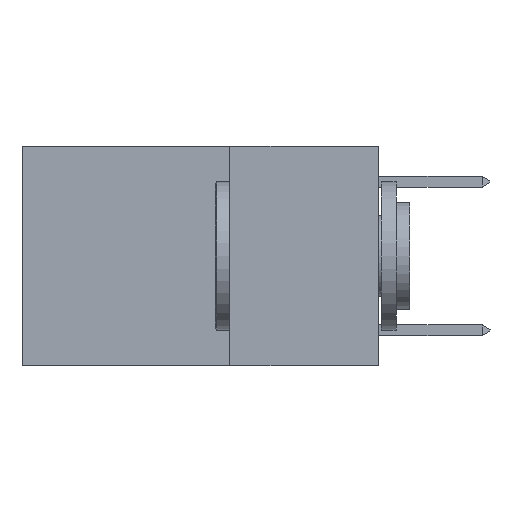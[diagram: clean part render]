
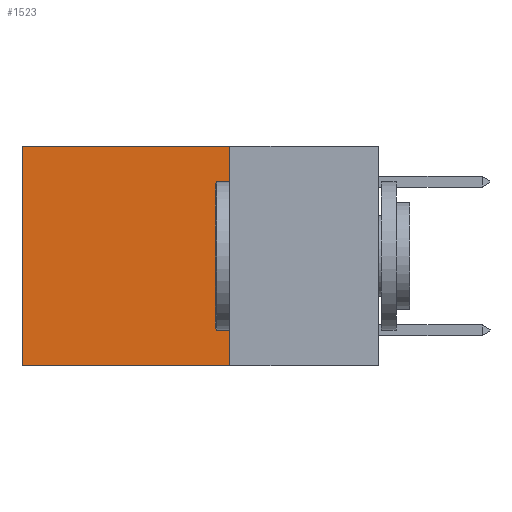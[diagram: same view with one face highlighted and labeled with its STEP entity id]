
A CAD part, left-side view. The second image highlights one B-rep face of the part: STEP entity #1523.
In plain terms, the highlighted planar face has unit normal (-1, 0, 0).
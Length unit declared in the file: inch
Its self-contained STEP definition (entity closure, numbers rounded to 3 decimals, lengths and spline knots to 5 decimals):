
#1523 = ADVANCED_FACE ( 'NONE', ( #4205 ), #27941, .F. ) ;
#2537 = CARTESIAN_POINT ( 'NONE',  ( 0.2625, 0.6, 0. ) ) ;
#2686 = DIRECTION ( 'NONE',  ( 0., 1., 0. ) ) ;
#3125 = EDGE_CURVE ( 'NONE', #14045, #5056, #6035, .T. ) ;
#4205 = FACE_OUTER_BOUND ( 'NONE', #26164, .T. ) ;
#5056 = VERTEX_POINT ( 'NONE', #5324 ) ;
#5106 = VECTOR ( 'NONE', #6138, 39.37008 ) ;
#5324 = CARTESIAN_POINT ( 'NONE',  ( 0.2625, 0.25, -0.37 ) ) ;
#6035 = LINE ( 'NONE', #10715, #5106 ) ;
#6131 = DIRECTION ( 'NONE',  ( 0., 0., -1. ) ) ;
#6138 = DIRECTION ( 'NONE',  ( 0., 0., -1. ) ) ;
#8588 = CARTESIAN_POINT ( 'NONE',  ( 0.2625, 0.25, 0. ) ) ;
#9361 = LINE ( 'NONE', #8588, #15539 ) ;
#10715 = CARTESIAN_POINT ( 'NONE',  ( 0.2625, 0.25, 0. ) ) ;
#11117 = AXIS2_PLACEMENT_3D ( 'NONE', #27568, #27295, #27123 ) ;
#11967 = CARTESIAN_POINT ( 'NONE',  ( 0.2625, 0.25, -0.37 ) ) ;
#13544 = EDGE_CURVE ( 'NONE', #5056, #22666, #13981, .T. ) ;
#13766 = VECTOR ( 'NONE', #2686, 39.37008 ) ;
#13981 = LINE ( 'NONE', #11967, #13766 ) ;
#14045 = VERTEX_POINT ( 'NONE', #25362 ) ;
#14818 = ORIENTED_EDGE ( 'NONE', *, *, #15388, .T. ) ;
#15388 = EDGE_CURVE ( 'NONE', #28329, #22666, #28771, .T. ) ;
#15463 = CARTESIAN_POINT ( 'NONE',  ( 0.2625, 0.6, 0. ) ) ;
#15539 = VECTOR ( 'NONE', #20154, 39.37008 ) ;
#19988 = ORIENTED_EDGE ( 'NONE', *, *, #13544, .F. ) ;
#20154 = DIRECTION ( 'NONE',  ( 0., 1., 0. ) ) ;
#22666 = VERTEX_POINT ( 'NONE', #28288 ) ;
#22714 = ORIENTED_EDGE ( 'NONE', *, *, #24795, .T. ) ;
#24795 = EDGE_CURVE ( 'NONE', #14045, #28329, #9361, .T. ) ;
#25248 = ORIENTED_EDGE ( 'NONE', *, *, #3125, .F. ) ;
#25362 = CARTESIAN_POINT ( 'NONE',  ( 0.2625, 0.25, 0. ) ) ;
#26164 = EDGE_LOOP ( 'NONE', ( #14818, #19988, #25248, #22714 ) ) ;
#27123 = DIRECTION ( 'NONE',  ( 0., 0., -1. ) ) ;
#27295 = DIRECTION ( 'NONE',  ( 1., 0., 0. ) ) ;
#27568 = CARTESIAN_POINT ( 'NONE',  ( 0.2625, 0.25, 0. ) ) ;
#27941 = PLANE ( 'NONE',  #11117 ) ;
#28288 = CARTESIAN_POINT ( 'NONE',  ( 0.2625, 0.6, -0.37 ) ) ;
#28329 = VERTEX_POINT ( 'NONE', #2537 ) ;
#28771 = LINE ( 'NONE', #15463, #28801 ) ;
#28801 = VECTOR ( 'NONE', #6131, 39.37008 ) ;
